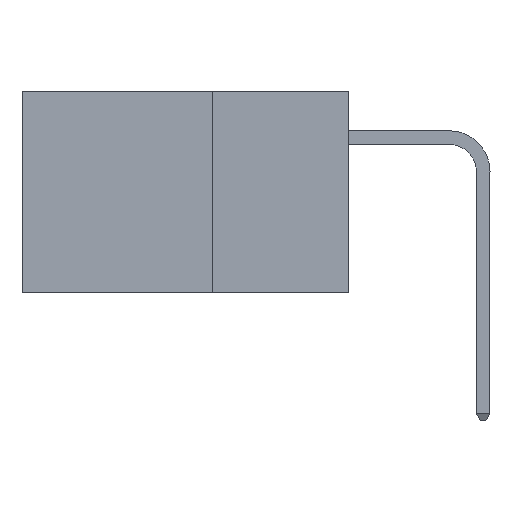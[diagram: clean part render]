
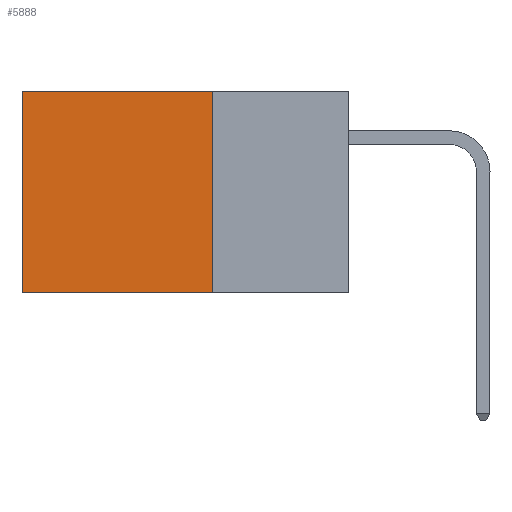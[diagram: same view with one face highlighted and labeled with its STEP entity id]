
A CAD part, left-side view. The second image highlights one B-rep face of the part: STEP entity #5888.
In plain terms, the highlighted planar face has unit normal (-1, 0, 0).
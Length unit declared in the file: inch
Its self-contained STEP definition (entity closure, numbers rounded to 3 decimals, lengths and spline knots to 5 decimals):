
#100 = CARTESIAN_POINT ( 'NONE',  ( 0.2875, 0.25, 0. ) ) ;
#418 = CARTESIAN_POINT ( 'NONE',  ( 0.2875, 0.25, -0.37 ) ) ;
#822 = ORIENTED_EDGE ( 'NONE', *, *, #5185, .F. ) ;
#890 = VECTOR ( 'NONE', #8212, 39.37008 ) ;
#1125 = LINE ( 'NONE', #418, #890 ) ;
#1927 = VERTEX_POINT ( 'NONE', #6647 ) ;
#2059 = CARTESIAN_POINT ( 'NONE',  ( 0.2875, 0.25, -0.37 ) ) ;
#2311 = VECTOR ( 'NONE', #7809, 39.37008 ) ;
#2317 = LINE ( 'NONE', #7653, #2311 ) ;
#3083 = LINE ( 'NONE', #8530, #5052 ) ;
#3100 = DIRECTION ( 'NONE',  ( 0., 0., -1. ) ) ;
#4331 = VERTEX_POINT ( 'NONE', #2059 ) ;
#4579 = ORIENTED_EDGE ( 'NONE', *, *, #8745, .T. ) ;
#4715 = VECTOR ( 'NONE', #9173, 39.37008 ) ;
#5052 = VECTOR ( 'NONE', #9225, 39.37008 ) ;
#5185 = EDGE_CURVE ( 'NONE', #4331, #1927, #1125, .T. ) ;
#5888 = ADVANCED_FACE ( 'NONE', ( #7893 ), #8631, .F. ) ;
#6203 = ORIENTED_EDGE ( 'NONE', *, *, #8989, .F. ) ;
#6241 = DIRECTION ( 'NONE',  ( 1., 0., 0. ) ) ;
#6302 = EDGE_CURVE ( 'NONE', #8097, #9579, #3083, .T. ) ;
#6623 = CARTESIAN_POINT ( 'NONE',  ( 0.2875, 0.25, 0. ) ) ;
#6647 = CARTESIAN_POINT ( 'NONE',  ( 0.2875, 0.6, -0.37 ) ) ;
#6882 = EDGE_LOOP ( 'NONE', ( #4579, #822, #6203, #8993 ) ) ;
#7653 = CARTESIAN_POINT ( 'NONE',  ( 0.2875, 0.6, 0. ) ) ;
#7770 = CARTESIAN_POINT ( 'NONE',  ( 0.2875, 0.6, 0. ) ) ;
#7809 = DIRECTION ( 'NONE',  ( 0., 0., -1. ) ) ;
#7893 = FACE_OUTER_BOUND ( 'NONE', #6882, .T. ) ;
#8097 = VERTEX_POINT ( 'NONE', #6623 ) ;
#8212 = DIRECTION ( 'NONE',  ( 0., 1., 0. ) ) ;
#8472 = LINE ( 'NONE', #9831, #4715 ) ;
#8530 = CARTESIAN_POINT ( 'NONE',  ( 0.2875, 0.25, 0. ) ) ;
#8631 = PLANE ( 'NONE',  #9182 ) ;
#8745 = EDGE_CURVE ( 'NONE', #9579, #1927, #2317, .T. ) ;
#8989 = EDGE_CURVE ( 'NONE', #8097, #4331, #8472, .T. ) ;
#8993 = ORIENTED_EDGE ( 'NONE', *, *, #6302, .T. ) ;
#9173 = DIRECTION ( 'NONE',  ( 0., 0., -1. ) ) ;
#9182 = AXIS2_PLACEMENT_3D ( 'NONE', #100, #6241, #3100 ) ;
#9225 = DIRECTION ( 'NONE',  ( 0., 1., 0. ) ) ;
#9579 = VERTEX_POINT ( 'NONE', #7770 ) ;
#9831 = CARTESIAN_POINT ( 'NONE',  ( 0.2875, 0.25, 0. ) ) ;
